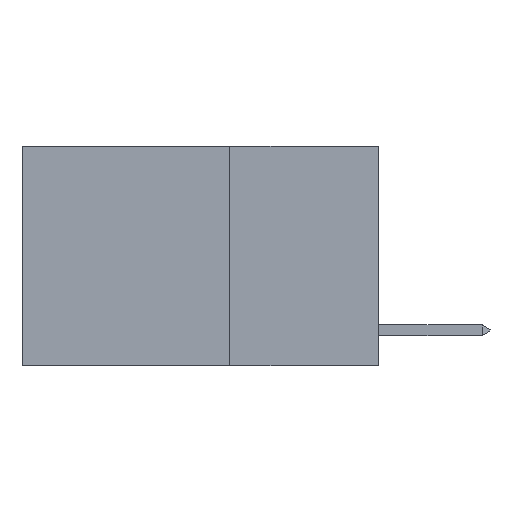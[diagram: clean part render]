
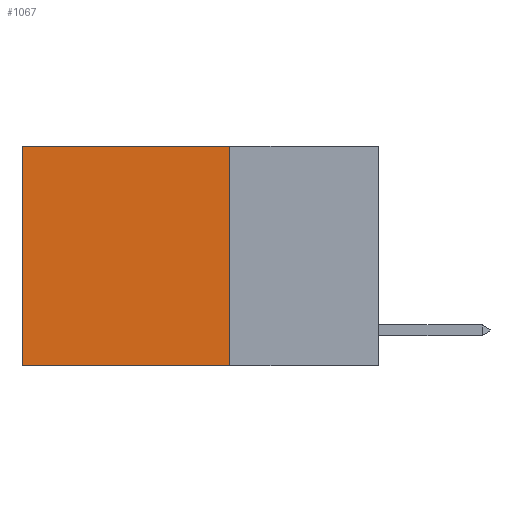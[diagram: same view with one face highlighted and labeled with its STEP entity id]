
A CAD part, left-side view. The second image highlights one B-rep face of the part: STEP entity #1067.
In plain terms, the highlighted planar face has unit normal (-1, 0, 0).
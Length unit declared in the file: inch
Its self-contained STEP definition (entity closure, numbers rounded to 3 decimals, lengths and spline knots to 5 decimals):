
#413 = DIRECTION ( 'NONE',  ( 0., 1., 0. ) ) ;
#637 = VERTEX_POINT ( 'NONE', #8268 ) ;
#768 = EDGE_CURVE ( 'NONE', #6579, #637, #10211, .T. ) ;
#904 = VECTOR ( 'NONE', #1660, 39.37008 ) ;
#933 = ORIENTED_EDGE ( 'NONE', *, *, #9159, .T. ) ;
#1067 = ADVANCED_FACE ( 'NONE', ( #3055 ), #9899, .F. ) ;
#1089 = CARTESIAN_POINT ( 'NONE',  ( 0.2625, 0.25, -0.37 ) ) ;
#1660 = DIRECTION ( 'NONE',  ( 0., 0., -1. ) ) ;
#2143 = LINE ( 'NONE', #10385, #4804 ) ;
#2193 = CARTESIAN_POINT ( 'NONE',  ( 0.2625, 0.25, 0. ) ) ;
#2891 = VECTOR ( 'NONE', #7969, 39.37008 ) ;
#2909 = DIRECTION ( 'NONE',  ( 0., 1., 0. ) ) ;
#3055 = FACE_OUTER_BOUND ( 'NONE', #5259, .T. ) ;
#3468 = VECTOR ( 'NONE', #2909, 39.37008 ) ;
#4528 = AXIS2_PLACEMENT_3D ( 'NONE', #2193, #5484, #6383 ) ;
#4540 = CARTESIAN_POINT ( 'NONE',  ( 0.2625, 0.25, 0. ) ) ;
#4728 = ORIENTED_EDGE ( 'NONE', *, *, #5583, .F. ) ;
#4804 = VECTOR ( 'NONE', #413, 39.37008 ) ;
#4942 = ORIENTED_EDGE ( 'NONE', *, *, #768, .T. ) ;
#5259 = EDGE_LOOP ( 'NONE', ( #4942, #4728, #8936, #933 ) ) ;
#5484 = DIRECTION ( 'NONE',  ( 1., 0., 0. ) ) ;
#5583 = EDGE_CURVE ( 'NONE', #8728, #637, #2143, .T. ) ;
#6330 = LINE ( 'NONE', #4540, #2891 ) ;
#6357 = CARTESIAN_POINT ( 'NONE',  ( 0.2625, 0.25, 0. ) ) ;
#6383 = DIRECTION ( 'NONE',  ( 0., 0., -1. ) ) ;
#6579 = VERTEX_POINT ( 'NONE', #7524 ) ;
#7312 = EDGE_CURVE ( 'NONE', #8489, #8728, #6330, .T. ) ;
#7524 = CARTESIAN_POINT ( 'NONE',  ( 0.2625, 0.6, 0. ) ) ;
#7969 = DIRECTION ( 'NONE',  ( 0., 0., -1. ) ) ;
#8268 = CARTESIAN_POINT ( 'NONE',  ( 0.2625, 0.6, -0.37 ) ) ;
#8489 = VERTEX_POINT ( 'NONE', #9583 ) ;
#8728 = VERTEX_POINT ( 'NONE', #1089 ) ;
#8936 = ORIENTED_EDGE ( 'NONE', *, *, #7312, .F. ) ;
#9159 = EDGE_CURVE ( 'NONE', #8489, #6579, #10407, .T. ) ;
#9250 = CARTESIAN_POINT ( 'NONE',  ( 0.2625, 0.6, 0. ) ) ;
#9583 = CARTESIAN_POINT ( 'NONE',  ( 0.2625, 0.25, 0. ) ) ;
#9899 = PLANE ( 'NONE',  #4528 ) ;
#10211 = LINE ( 'NONE', #9250, #904 ) ;
#10385 = CARTESIAN_POINT ( 'NONE',  ( 0.2625, 0.25, -0.37 ) ) ;
#10407 = LINE ( 'NONE', #6357, #3468 ) ;
